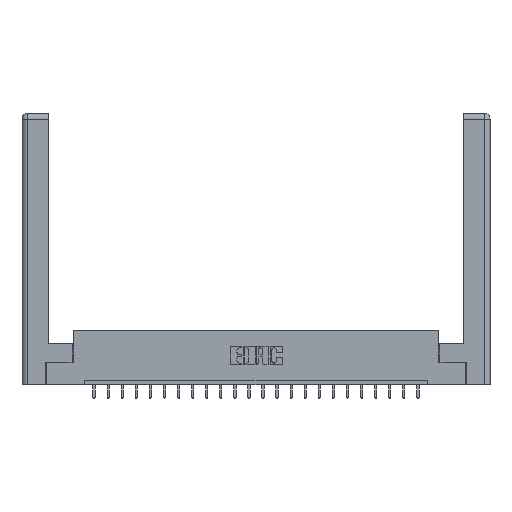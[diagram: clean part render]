
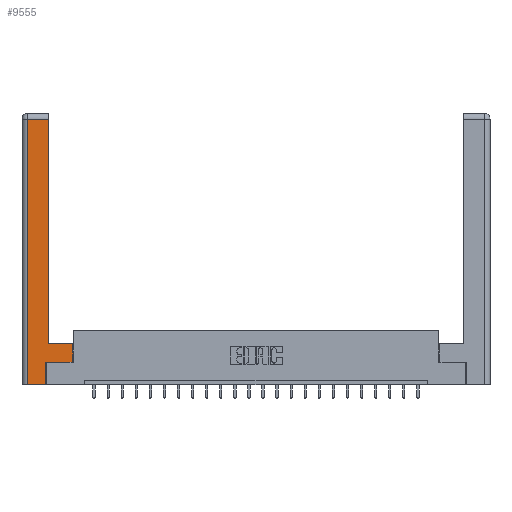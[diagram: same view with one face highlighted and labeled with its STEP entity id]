
A CAD part, top view. The second image highlights one B-rep face of the part: STEP entity #9555.
In plain terms, the highlighted planar face has unit normal (0, 0, 1).
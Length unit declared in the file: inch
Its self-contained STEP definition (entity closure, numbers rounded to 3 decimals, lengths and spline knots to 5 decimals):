
#46 = VECTOR ( 'NONE', #12428, 39.37008 ) ;
#209 = CARTESIAN_POINT ( 'NONE',  ( 0.0615, 2.94, 0. ) ) ;
#405 = CARTESIAN_POINT ( 'NONE',  ( 0.265, 0., 0. ) ) ;
#771 = DIRECTION ( 'NONE',  ( 0., 1., 0. ) ) ;
#962 = ORIENTED_EDGE ( 'NONE', *, *, #8431, .T. ) ;
#1369 = VECTOR ( 'NONE', #18452, 39.37008 ) ;
#1626 = DIRECTION ( 'NONE',  ( 1., 0., 0. ) ) ;
#2710 = CARTESIAN_POINT ( 'NONE',  ( 0., 0., 0. ) ) ;
#3156 = CARTESIAN_POINT ( 'NONE',  ( 0.565, 0.245, 0. ) ) ;
#3158 = VECTOR ( 'NONE', #8223, 39.37008 ) ;
#3361 = CARTESIAN_POINT ( 'NONE',  ( 0.295, 0.45, 0. ) ) ;
#4801 = CARTESIAN_POINT ( 'NONE',  ( 0.565, 0.45, 0. ) ) ;
#4814 = CARTESIAN_POINT ( 'NONE',  ( 0.295, 2.94, 0. ) ) ;
#4960 = VECTOR ( 'NONE', #6943, 39.37008 ) ;
#5294 = VERTEX_POINT ( 'NONE', #21457 ) ;
#5380 = VECTOR ( 'NONE', #18962, 39.37008 ) ;
#5571 = EDGE_CURVE ( 'NONE', #16333, #11587, #19138, .T. ) ;
#5719 = EDGE_CURVE ( 'NONE', #11587, #12816, #12512, .T. ) ;
#6316 = CARTESIAN_POINT ( 'NONE',  ( 0.565, 0.245, 0. ) ) ;
#6943 = DIRECTION ( 'NONE',  ( 0., -1., 0. ) ) ;
#6957 = VECTOR ( 'NONE', #1626, 39.37008 ) ;
#7118 = DIRECTION ( 'NONE',  ( -1., 0., 0. ) ) ;
#7515 = LINE ( 'NONE', #14786, #14403 ) ;
#7548 = CARTESIAN_POINT ( 'NONE',  ( 0.265, 0.245, 0. ) ) ;
#8172 = EDGE_CURVE ( 'NONE', #18332, #16383, #16549, .T. ) ;
#8223 = DIRECTION ( 'NONE',  ( 0., 1., 0. ) ) ;
#8431 = EDGE_CURVE ( 'NONE', #12563, #16333, #20129, .T. ) ;
#8700 = CARTESIAN_POINT ( 'NONE',  ( 0.0615, 0., 0. ) ) ;
#9359 = ORIENTED_EDGE ( 'NONE', *, *, #11364, .T. ) ;
#9363 = ORIENTED_EDGE ( 'NONE', *, *, #10372, .T. ) ;
#9375 = LINE ( 'NONE', #3361, #46 ) ;
#9555 = ADVANCED_FACE ( 'NONE', ( #21918 ), #11836, .F. ) ;
#9845 = DIRECTION ( 'NONE',  ( 0., 0., -1. ) ) ;
#10372 = EDGE_CURVE ( 'NONE', #5294, #19612, #7515, .T. ) ;
#10490 = EDGE_LOOP ( 'NONE', ( #9363, #9359, #20295, #13452, #962, #19671, #12045, #17859 ) ) ;
#11024 = AXIS2_PLACEMENT_3D ( 'NONE', #2710, #9845, #22199 ) ;
#11364 = EDGE_CURVE ( 'NONE', #19612, #18332, #12435, .T. ) ;
#11587 = VERTEX_POINT ( 'NONE', #6316 ) ;
#11836 = PLANE ( 'NONE',  #11024 ) ;
#12045 = ORIENTED_EDGE ( 'NONE', *, *, #5719, .T. ) ;
#12146 = CARTESIAN_POINT ( 'NONE',  ( 0.265, 0., 0. ) ) ;
#12428 = DIRECTION ( 'NONE',  ( -1., 0., 0. ) ) ;
#12435 = LINE ( 'NONE', #209, #19938 ) ;
#12512 = LINE ( 'NONE', #4801, #3158 ) ;
#12563 = VERTEX_POINT ( 'NONE', #405 ) ;
#12816 = VERTEX_POINT ( 'NONE', #16098 ) ;
#13452 = ORIENTED_EDGE ( 'NONE', *, *, #18418, .T. ) ;
#14403 = VECTOR ( 'NONE', #771, 39.37008 ) ;
#14709 = LINE ( 'NONE', #12146, #6957 ) ;
#14786 = CARTESIAN_POINT ( 'NONE',  ( 0.295, 3., 0. ) ) ;
#15471 = CARTESIAN_POINT ( 'NONE',  ( 0.0615, 2.94, 0. ) ) ;
#16098 = CARTESIAN_POINT ( 'NONE',  ( 0.565, 0.45, 0. ) ) ;
#16333 = VERTEX_POINT ( 'NONE', #7548 ) ;
#16383 = VERTEX_POINT ( 'NONE', #18585 ) ;
#16549 = LINE ( 'NONE', #8700, #4960 ) ;
#17859 = ORIENTED_EDGE ( 'NONE', *, *, #21545, .T. ) ;
#18332 = VERTEX_POINT ( 'NONE', #15471 ) ;
#18418 = EDGE_CURVE ( 'NONE', #16383, #12563, #14709, .T. ) ;
#18452 = DIRECTION ( 'NONE',  ( 0., 1., 0. ) ) ;
#18585 = CARTESIAN_POINT ( 'NONE',  ( 0.0615, 0., 0. ) ) ;
#18962 = DIRECTION ( 'NONE',  ( 1., 0., 0. ) ) ;
#19138 = LINE ( 'NONE', #3156, #5380 ) ;
#19612 = VERTEX_POINT ( 'NONE', #4814 ) ;
#19671 = ORIENTED_EDGE ( 'NONE', *, *, #5571, .T. ) ;
#19919 = CARTESIAN_POINT ( 'NONE',  ( 0.265, 0.245, 0. ) ) ;
#19938 = VECTOR ( 'NONE', #7118, 39.37008 ) ;
#20129 = LINE ( 'NONE', #19919, #1369 ) ;
#20295 = ORIENTED_EDGE ( 'NONE', *, *, #8172, .T. ) ;
#21457 = CARTESIAN_POINT ( 'NONE',  ( 0.295, 0.45, 0. ) ) ;
#21545 = EDGE_CURVE ( 'NONE', #12816, #5294, #9375, .T. ) ;
#21918 = FACE_OUTER_BOUND ( 'NONE', #10490, .T. ) ;
#22199 = DIRECTION ( 'NONE',  ( -1., 0., 0. ) ) ;
